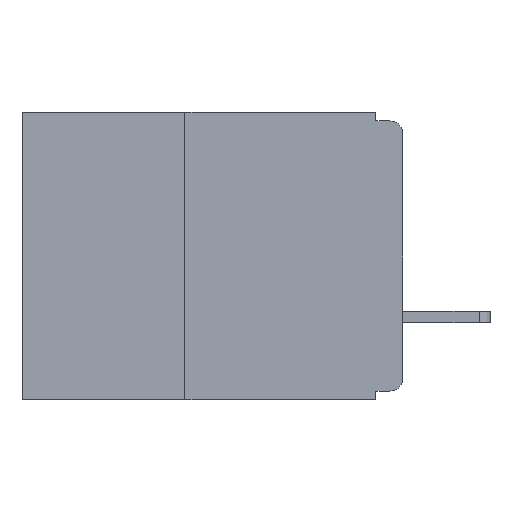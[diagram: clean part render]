
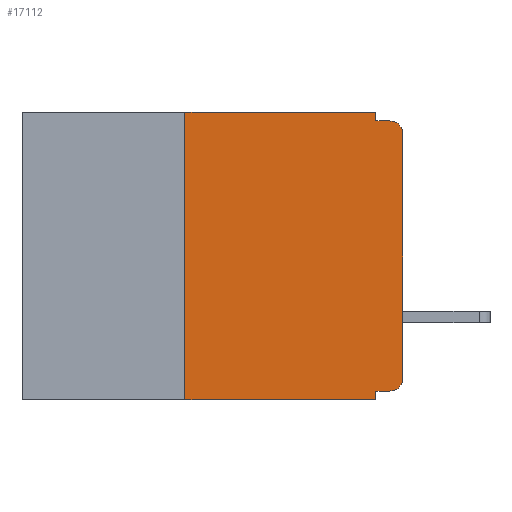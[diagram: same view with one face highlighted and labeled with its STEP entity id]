
A CAD part, left-side view. The second image highlights one B-rep face of the part: STEP entity #17112.
In plain terms, the highlighted planar face has unit normal (-1, 0, 0).
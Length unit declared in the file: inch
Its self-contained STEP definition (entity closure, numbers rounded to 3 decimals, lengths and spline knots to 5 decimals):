
#483 = CARTESIAN_POINT ( 'NONE',  ( 0., 0., -0.025 ) ) ;
#850 = PLANE ( 'NONE',  #1349 ) ;
#1331 = CARTESIAN_POINT ( 'NONE',  ( 0., 0.031, -0.33 ) ) ;
#1349 = AXIS2_PLACEMENT_3D ( 'NONE', #13817, #3063, #18129 ) ;
#1364 = CARTESIAN_POINT ( 'NONE',  ( 0., 0.031, -0.33 ) ) ;
#1970 = CARTESIAN_POINT ( 'NONE',  ( 0., 0.031, 0. ) ) ;
#3063 = DIRECTION ( 'NONE',  ( 1., 0., 0. ) ) ;
#3119 = DIRECTION ( 'NONE',  ( 0., 0., 1. ) ) ;
#3755 = EDGE_CURVE ( 'NONE', #11010, #13959, #26573, .T. ) ;
#4844 = VECTOR ( 'NONE', #18626, 39.37008 ) ;
#4960 = VERTEX_POINT ( 'NONE', #18794 ) ;
#5421 = VECTOR ( 'NONE', #17757, 39.37008 ) ;
#6205 = DIRECTION ( 'NONE',  ( 0., 1., 0. ) ) ;
#6333 = ORIENTED_EDGE ( 'NONE', *, *, #9615, .T. ) ;
#6349 = DIRECTION ( 'NONE',  ( 0., 0., -1. ) ) ;
#6669 = CARTESIAN_POINT ( 'NONE',  ( 0., 0.25, -0.33 ) ) ;
#6747 = VERTEX_POINT ( 'NONE', #483 ) ;
#8414 = CIRCLE ( 'NONE', #14056, 0.015 ) ;
#8442 = ORIENTED_EDGE ( 'NONE', *, *, #11930, .F. ) ;
#8504 = DIRECTION ( 'NONE',  ( -1., 0., 0. ) ) ;
#8611 = CARTESIAN_POINT ( 'NONE',  ( 0., 0.437, -0.33 ) ) ;
#8680 = ORIENTED_EDGE ( 'NONE', *, *, #15672, .F. ) ;
#8804 = CARTESIAN_POINT ( 'NONE',  ( 0., 0.015, -0.32 ) ) ;
#9517 = ORIENTED_EDGE ( 'NONE', *, *, #22424, .F. ) ;
#9615 = EDGE_CURVE ( 'NONE', #6747, #27419, #8414, .T. ) ;
#9622 = VERTEX_POINT ( 'NONE', #19174 ) ;
#9866 = LINE ( 'NONE', #13881, #21220 ) ;
#9924 = VECTOR ( 'NONE', #6205, 39.37008 ) ;
#10540 = LINE ( 'NONE', #1970, #15569 ) ;
#11010 = VERTEX_POINT ( 'NONE', #8804 ) ;
#11369 = EDGE_CURVE ( 'NONE', #24501, #26576, #21944, .T. ) ;
#11930 = EDGE_CURVE ( 'NONE', #4960, #27419, #14274, .T. ) ;
#12812 = EDGE_CURVE ( 'NONE', #26847, #26576, #13927, .T. ) ;
#13196 = EDGE_LOOP ( 'NONE', ( #26627, #6333, #8442, #24782, #17869, #8680, #27174, #16964, #9517, #27673 ) ) ;
#13434 = CARTESIAN_POINT ( 'NONE',  ( 0., 0.25, -0.33 ) ) ;
#13550 = CARTESIAN_POINT ( 'NONE',  ( 0., 0.031, -0.32 ) ) ;
#13606 = VECTOR ( 'NONE', #26685, 39.37008 ) ;
#13817 = CARTESIAN_POINT ( 'NONE',  ( 0., 0.437, 0. ) ) ;
#13881 = CARTESIAN_POINT ( 'NONE',  ( 0., 0., 0. ) ) ;
#13927 = LINE ( 'NONE', #8611, #24505 ) ;
#13959 = VERTEX_POINT ( 'NONE', #24264 ) ;
#14056 = AXIS2_PLACEMENT_3D ( 'NONE', #21290, #8504, #23380 ) ;
#14086 = DIRECTION ( 'NONE',  ( 0., 0., -1. ) ) ;
#14114 = DIRECTION ( 'NONE',  ( -1., 0., 0. ) ) ;
#14140 = CARTESIAN_POINT ( 'NONE',  ( 0., 0.015, -0.305 ) ) ;
#14274 = LINE ( 'NONE', #22606, #13606 ) ;
#14706 = VERTEX_POINT ( 'NONE', #26558 ) ;
#15569 = VECTOR ( 'NONE', #6349, 39.37008 ) ;
#15616 = LINE ( 'NONE', #21180, #9924 ) ;
#15656 = AXIS2_PLACEMENT_3D ( 'NONE', #14140, #14114, #14086 ) ;
#15672 = EDGE_CURVE ( 'NONE', #26847, #14706, #17551, .T. ) ;
#15968 = CARTESIAN_POINT ( 'NONE',  ( 0., 0.437, 0. ) ) ;
#16073 = DIRECTION ( 'NONE',  ( 0., -1., 0. ) ) ;
#16964 = ORIENTED_EDGE ( 'NONE', *, *, #11369, .F. ) ;
#17112 = ADVANCED_FACE ( 'NONE', ( #24675 ), #850, .F. ) ;
#17551 = LINE ( 'NONE', #13434, #5421 ) ;
#17757 = DIRECTION ( 'NONE',  ( 0., 0., 1. ) ) ;
#17869 = ORIENTED_EDGE ( 'NONE', *, *, #20448, .F. ) ;
#18129 = DIRECTION ( 'NONE',  ( 0., 0., -1. ) ) ;
#18626 = DIRECTION ( 'NONE',  ( 0., 0., -1. ) ) ;
#18794 = CARTESIAN_POINT ( 'NONE',  ( 0., 0.031, -0.01 ) ) ;
#19174 = CARTESIAN_POINT ( 'NONE',  ( 0., 0.031, 0. ) ) ;
#20448 = EDGE_CURVE ( 'NONE', #14706, #9622, #25453, .T. ) ;
#20586 = VECTOR ( 'NONE', #16073, 39.37008 ) ;
#21180 = CARTESIAN_POINT ( 'NONE',  ( 0., 0., -0.32 ) ) ;
#21220 = VECTOR ( 'NONE', #3119, 39.37008 ) ;
#21290 = CARTESIAN_POINT ( 'NONE',  ( 0., 0.015, -0.025 ) ) ;
#21385 = EDGE_CURVE ( 'NONE', #9622, #4960, #10540, .T. ) ;
#21816 = CARTESIAN_POINT ( 'NONE',  ( 0., 0.015, -0.01 ) ) ;
#21944 = LINE ( 'NONE', #1364, #4844 ) ;
#22424 = EDGE_CURVE ( 'NONE', #11010, #24501, #15616, .T. ) ;
#22606 = CARTESIAN_POINT ( 'NONE',  ( 0., 0., -0.01 ) ) ;
#23325 = EDGE_CURVE ( 'NONE', #13959, #6747, #9866, .T. ) ;
#23380 = DIRECTION ( 'NONE',  ( 0., 0., -1. ) ) ;
#23495 = DIRECTION ( 'NONE',  ( 0., -1., 0. ) ) ;
#24264 = CARTESIAN_POINT ( 'NONE',  ( 0., 0., -0.305 ) ) ;
#24501 = VERTEX_POINT ( 'NONE', #13550 ) ;
#24505 = VECTOR ( 'NONE', #23495, 39.37008 ) ;
#24675 = FACE_OUTER_BOUND ( 'NONE', #13196, .T. ) ;
#24782 = ORIENTED_EDGE ( 'NONE', *, *, #21385, .F. ) ;
#25453 = LINE ( 'NONE', #15968, #20586 ) ;
#26558 = CARTESIAN_POINT ( 'NONE',  ( 0., 0.25, 0. ) ) ;
#26573 = CIRCLE ( 'NONE', #15656, 0.015 ) ;
#26576 = VERTEX_POINT ( 'NONE', #1331 ) ;
#26627 = ORIENTED_EDGE ( 'NONE', *, *, #23325, .T. ) ;
#26685 = DIRECTION ( 'NONE',  ( 0., -1., 0. ) ) ;
#26847 = VERTEX_POINT ( 'NONE', #6669 ) ;
#27174 = ORIENTED_EDGE ( 'NONE', *, *, #12812, .T. ) ;
#27419 = VERTEX_POINT ( 'NONE', #21816 ) ;
#27673 = ORIENTED_EDGE ( 'NONE', *, *, #3755, .T. ) ;
